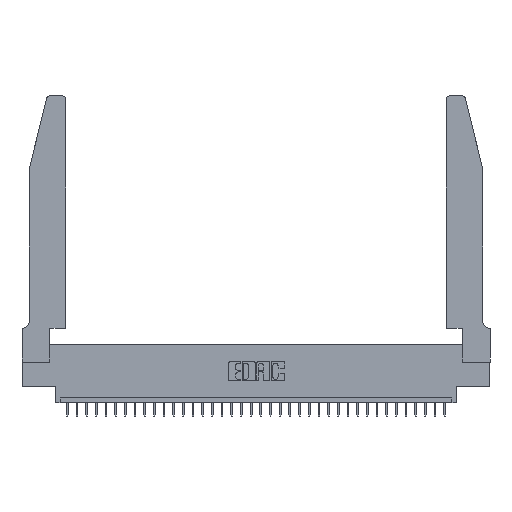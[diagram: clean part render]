
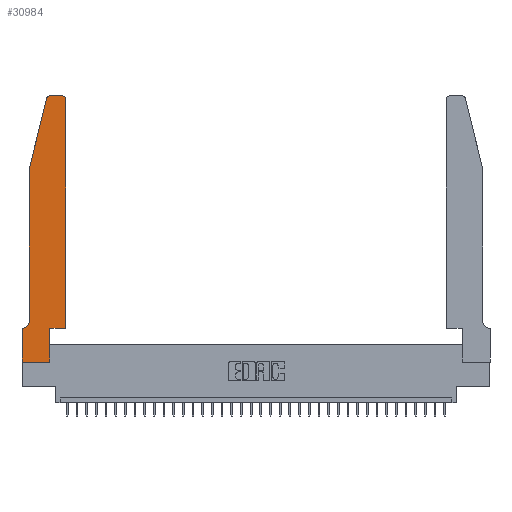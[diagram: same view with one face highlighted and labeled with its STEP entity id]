
A CAD part, top view. The second image highlights one B-rep face of the part: STEP entity #30984.
In plain terms, the highlighted planar face has unit normal (0, 0, 1).
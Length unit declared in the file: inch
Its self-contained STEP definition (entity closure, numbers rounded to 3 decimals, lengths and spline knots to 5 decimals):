
#346 = ORIENTED_EDGE ( 'NONE', *, *, #20064, .T. ) ;
#832 = AXIS2_PLACEMENT_3D ( 'NONE', #30744, #8594, #25024 ) ;
#865 = AXIS2_PLACEMENT_3D ( 'NONE', #31281, #33441, #6813 ) ;
#878 = LINE ( 'NONE', #11939, #5765 ) ;
#977 = CARTESIAN_POINT ( 'NONE',  ( 0.2605, 2.75, 0.37 ) ) ;
#1093 = DIRECTION ( 'NONE',  ( 1., 0., 0. ) ) ;
#1458 = LINE ( 'NONE', #28444, #6124 ) ;
#1527 = ORIENTED_EDGE ( 'NONE', *, *, #19512, .T. ) ;
#2180 = EDGE_CURVE ( 'NONE', #10250, #29090, #9853, .T. ) ;
#2299 = ORIENTED_EDGE ( 'NONE', *, *, #22376, .T. ) ;
#2964 = ORIENTED_EDGE ( 'NONE', *, *, #17318, .T. ) ;
#3448 = CIRCLE ( 'NONE', #13127, 0.03 ) ;
#3522 = ORIENTED_EDGE ( 'NONE', *, *, #6969, .T. ) ;
#3722 = VECTOR ( 'NONE', #14893, 39.37008 ) ;
#4305 = CARTESIAN_POINT ( 'NONE',  ( 0.284, 2.72, 0.37 ) ) ;
#4383 = DIRECTION ( 'NONE',  ( 0., 0., 1. ) ) ;
#4688 = DIRECTION ( 'NONE',  ( 0., -1., 0. ) ) ;
#4863 = VERTEX_POINT ( 'NONE', #27689 ) ;
#5765 = VECTOR ( 'NONE', #17466, 39.37008 ) ;
#6124 = VECTOR ( 'NONE', #26297, 39.37008 ) ;
#6173 = LINE ( 'NONE', #32981, #33148 ) ;
#6506 = VERTEX_POINT ( 'NONE', #15857 ) ;
#6813 = DIRECTION ( 'NONE',  ( -1., 0., 0. ) ) ;
#6969 = EDGE_CURVE ( 'NONE', #7924, #4863, #6173, .T. ) ;
#7084 = VECTOR ( 'NONE', #10293, 39.37008 ) ;
#7270 = VERTEX_POINT ( 'NONE', #18267 ) ;
#7473 = CARTESIAN_POINT ( 'NONE',  ( 0.4205, 2.75, 0.37 ) ) ;
#7846 = VECTOR ( 'NONE', #31256, 39.37008 ) ;
#7924 = VERTEX_POINT ( 'NONE', #14914 ) ;
#8181 = ORIENTED_EDGE ( 'NONE', *, *, #12238, .T. ) ;
#8535 = VERTEX_POINT ( 'NONE', #29537 ) ;
#8563 = LINE ( 'NONE', #29421, #7084 ) ;
#8594 = DIRECTION ( 'NONE',  ( 0., 0., 1. ) ) ;
#9016 = LINE ( 'NONE', #977, #3722 ) ;
#9739 = DIRECTION ( 'NONE',  ( 1., 0., 0. ) ) ;
#9853 = LINE ( 'NONE', #16398, #11872 ) ;
#10250 = VERTEX_POINT ( 'NONE', #25014 ) ;
#10293 = DIRECTION ( 'NONE',  ( 1., 0., 0. ) ) ;
#10561 = VERTEX_POINT ( 'NONE', #7473 ) ;
#10852 = CIRCLE ( 'NONE', #15393, 0.03 ) ;
#11872 = VECTOR ( 'NONE', #4688, 39.37008 ) ;
#11939 = CARTESIAN_POINT ( 'NONE',  ( 0.4505, 0.35, 0.37 ) ) ;
#12238 = EDGE_CURVE ( 'NONE', #29090, #7924, #17954, .T. ) ;
#13127 = AXIS2_PLACEMENT_3D ( 'NONE', #4305, #25751, #1093 ) ;
#14809 = PLANE ( 'NONE',  #832 ) ;
#14818 = EDGE_CURVE ( 'NONE', #18541, #21582, #1458, .T. ) ;
#14893 = DIRECTION ( 'NONE',  ( -1., 0., 0. ) ) ;
#14914 = CARTESIAN_POINT ( 'NONE',  ( 0.0055, 0.35, 0.37 ) ) ;
#15393 = AXIS2_PLACEMENT_3D ( 'NONE', #23132, #4383, #9739 ) ;
#15449 = CARTESIAN_POINT ( 'NONE',  ( 0.2865, 0.35, 0.37 ) ) ;
#15857 = CARTESIAN_POINT ( 'NONE',  ( 0.4505, 0.35, 0.37 ) ) ;
#16398 = CARTESIAN_POINT ( 'NONE',  ( 0.0755, 2., 0.37 ) ) ;
#17305 = ORIENTED_EDGE ( 'NONE', *, *, #27748, .T. ) ;
#17318 = EDGE_CURVE ( 'NONE', #4863, #21048, #20359, .T. ) ;
#17466 = DIRECTION ( 'NONE',  ( 1., 0., 0. ) ) ;
#17720 = LINE ( 'NONE', #28287, #18905 ) ;
#17954 = CIRCLE ( 'NONE', #865, 0.07 ) ;
#18104 = CARTESIAN_POINT ( 'NONE',  ( 0.0755, 0.42, 0.37 ) ) ;
#18267 = CARTESIAN_POINT ( 'NONE',  ( 0.284, 2.75, 0.37 ) ) ;
#18541 = VERTEX_POINT ( 'NONE', #33459 ) ;
#18801 = ORIENTED_EDGE ( 'NONE', *, *, #2180, .T. ) ;
#18905 = VECTOR ( 'NONE', #28649, 39.37008 ) ;
#19284 = DIRECTION ( 'NONE',  ( 0., 1., 0. ) ) ;
#19512 = EDGE_CURVE ( 'NONE', #6506, #8535, #32874, .T. ) ;
#19851 = EDGE_LOOP ( 'NONE', ( #17305, #2299, #34564, #18801, #8181, #3522, #2964, #20330, #28666, #30561, #1527, #346 ) ) ;
#20032 = CARTESIAN_POINT ( 'NONE',  ( 0., 0., 0.37 ) ) ;
#20064 = EDGE_CURVE ( 'NONE', #8535, #10561, #10852, .T. ) ;
#20330 = ORIENTED_EDGE ( 'NONE', *, *, #26599, .T. ) ;
#20359 = LINE ( 'NONE', #28229, #7846 ) ;
#21048 = VERTEX_POINT ( 'NONE', #20032 ) ;
#21582 = VERTEX_POINT ( 'NONE', #15449 ) ;
#21958 = EDGE_CURVE ( 'NONE', #27904, #10250, #17720, .T. ) ;
#22376 = EDGE_CURVE ( 'NONE', #7270, #27904, #3448, .T. ) ;
#22692 = EDGE_CURVE ( 'NONE', #21582, #6506, #878, .T. ) ;
#23132 = CARTESIAN_POINT ( 'NONE',  ( 0.4205, 2.72, 0.37 ) ) ;
#23944 = VECTOR ( 'NONE', #19284, 39.37008 ) ;
#25014 = CARTESIAN_POINT ( 'NONE',  ( 0.0755, 2., 0.37 ) ) ;
#25024 = DIRECTION ( 'NONE',  ( 1., 0., 0. ) ) ;
#25751 = DIRECTION ( 'NONE',  ( 0., 0., 1. ) ) ;
#26297 = DIRECTION ( 'NONE',  ( 0., 1., 0. ) ) ;
#26599 = EDGE_CURVE ( 'NONE', #21048, #18541, #8563, .T. ) ;
#27689 = CARTESIAN_POINT ( 'NONE',  ( 0., 0.35, 0.37 ) ) ;
#27748 = EDGE_CURVE ( 'NONE', #10561, #7270, #9016, .T. ) ;
#27904 = VERTEX_POINT ( 'NONE', #32189 ) ;
#28229 = CARTESIAN_POINT ( 'NONE',  ( 0., 0., 0.37 ) ) ;
#28287 = CARTESIAN_POINT ( 'NONE',  ( 0.0755, 2., 0.37 ) ) ;
#28444 = CARTESIAN_POINT ( 'NONE',  ( 0.2865, 0.35, 0.37 ) ) ;
#28649 = DIRECTION ( 'NONE',  ( -0.239, -0.971, 0. ) ) ;
#28666 = ORIENTED_EDGE ( 'NONE', *, *, #14818, .T. ) ;
#29090 = VERTEX_POINT ( 'NONE', #18104 ) ;
#29421 = CARTESIAN_POINT ( 'NONE',  ( 0., 0., 0.37 ) ) ;
#29537 = CARTESIAN_POINT ( 'NONE',  ( 0.4505, 2.72, 0.37 ) ) ;
#30561 = ORIENTED_EDGE ( 'NONE', *, *, #22692, .T. ) ;
#30648 = DIRECTION ( 'NONE',  ( -1., 0., 0. ) ) ;
#30744 = CARTESIAN_POINT ( 'NONE',  ( 0., 0.35, 0.37 ) ) ;
#30984 = ADVANCED_FACE ( 'NONE', ( #33251 ), #14809, .T. ) ;
#31256 = DIRECTION ( 'NONE',  ( 0., -1., 0. ) ) ;
#31281 = CARTESIAN_POINT ( 'NONE',  ( 0.0055, 0.42, 0.37 ) ) ;
#32189 = CARTESIAN_POINT ( 'NONE',  ( 0.25487, 2.72718, 0.37 ) ) ;
#32874 = LINE ( 'NONE', #34709, #23944 ) ;
#32981 = CARTESIAN_POINT ( 'NONE',  ( 0.0755, 0.35, 0.37 ) ) ;
#33148 = VECTOR ( 'NONE', #30648, 39.37008 ) ;
#33251 = FACE_OUTER_BOUND ( 'NONE', #19851, .T. ) ;
#33441 = DIRECTION ( 'NONE',  ( 0., 0., -1. ) ) ;
#33459 = CARTESIAN_POINT ( 'NONE',  ( 0.2865, 0., 0.37 ) ) ;
#34564 = ORIENTED_EDGE ( 'NONE', *, *, #21958, .T. ) ;
#34709 = CARTESIAN_POINT ( 'NONE',  ( 0.4505, 0.35, 0.37 ) ) ;
